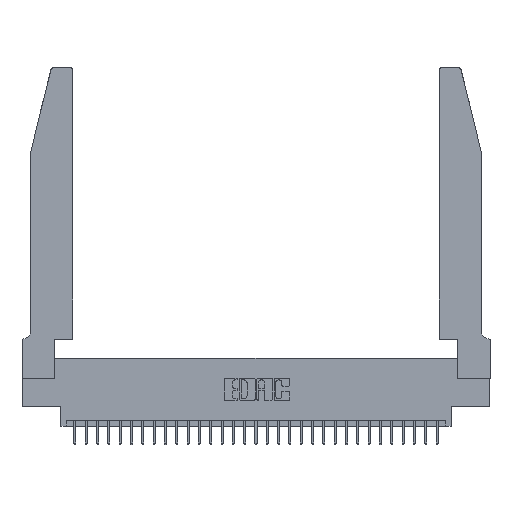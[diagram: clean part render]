
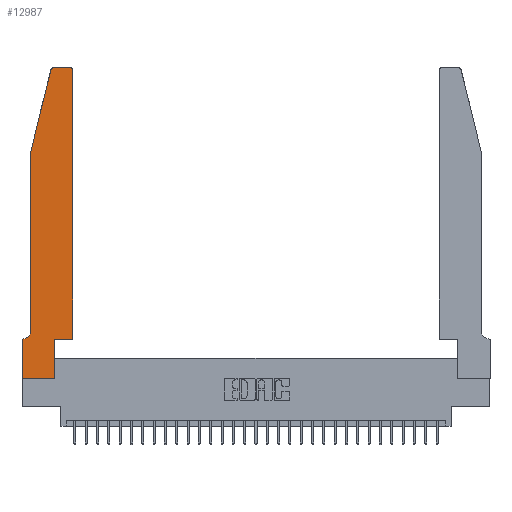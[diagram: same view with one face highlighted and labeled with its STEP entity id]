
A CAD part, top view. The second image highlights one B-rep face of the part: STEP entity #12987.
In plain terms, the highlighted planar face has unit normal (0, 0, 1).
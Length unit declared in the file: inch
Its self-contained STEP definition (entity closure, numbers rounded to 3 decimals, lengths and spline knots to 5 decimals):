
#38 = DIRECTION ( 'NONE',  ( 1., 0., 0. ) ) ;
#289 = EDGE_CURVE ( 'NONE', #4363, #17346, #24112, .T. ) ;
#447 = VERTEX_POINT ( 'NONE', #28399 ) ;
#587 = EDGE_LOOP ( 'NONE', ( #31960, #29077, #23572, #21709, #996, #9938, #24068, #21343, #4965, #27553, #31912, #23600 ) ) ;
#854 = VERTEX_POINT ( 'NONE', #930 ) ;
#930 = CARTESIAN_POINT ( 'NONE',  ( 0., 0.35, 0.37 ) ) ;
#996 = ORIENTED_EDGE ( 'NONE', *, *, #19184, .T. ) ;
#1919 = VERTEX_POINT ( 'NONE', #4878 ) ;
#2637 = CARTESIAN_POINT ( 'NONE',  ( 0.284, 2.72, 0.37 ) ) ;
#2673 = EDGE_CURVE ( 'NONE', #9499, #854, #15958, .T. ) ;
#2981 = CARTESIAN_POINT ( 'NONE',  ( 0.2865, 0.35, 0.37 ) ) ;
#3252 = CARTESIAN_POINT ( 'NONE',  ( 0.0755, 2., 0.37 ) ) ;
#4006 = CARTESIAN_POINT ( 'NONE',  ( 0.0755, 0.42, 0.37 ) ) ;
#4363 = VERTEX_POINT ( 'NONE', #11762 ) ;
#4402 = VECTOR ( 'NONE', #19186, 39.37008 ) ;
#4539 = LINE ( 'NONE', #12623, #24396 ) ;
#4878 = CARTESIAN_POINT ( 'NONE',  ( 0.284, 2.75, 0.37 ) ) ;
#4938 = CARTESIAN_POINT ( 'NONE',  ( 0.4505, 0.35, 0.37 ) ) ;
#4944 = CARTESIAN_POINT ( 'NONE',  ( 0., 0., 0.37 ) ) ;
#4965 = ORIENTED_EDGE ( 'NONE', *, *, #21294, .T. ) ;
#5196 = DIRECTION ( 'NONE',  ( 1., 0., 0. ) ) ;
#5439 = CARTESIAN_POINT ( 'NONE',  ( 0.25487, 2.72718, 0.37 ) ) ;
#5756 = VERTEX_POINT ( 'NONE', #14780 ) ;
#6135 = CIRCLE ( 'NONE', #13825, 0.03 ) ;
#6938 = EDGE_CURVE ( 'NONE', #13490, #1919, #31354, .T. ) ;
#6968 = VERTEX_POINT ( 'NONE', #4944 ) ;
#7221 = EDGE_CURVE ( 'NONE', #854, #6968, #30202, .T. ) ;
#7657 = LINE ( 'NONE', #10532, #20127 ) ;
#7766 = EDGE_CURVE ( 'NONE', #6968, #19508, #7657, .T. ) ;
#8386 = CARTESIAN_POINT ( 'NONE',  ( 0., 0., 0.37 ) ) ;
#8520 = VECTOR ( 'NONE', #12875, 39.37008 ) ;
#8575 = EDGE_CURVE ( 'NONE', #447, #13490, #12321, .T. ) ;
#8861 = CARTESIAN_POINT ( 'NONE',  ( 0.4205, 2.72, 0.37 ) ) ;
#9201 = CARTESIAN_POINT ( 'NONE',  ( 0.4505, 0.35, 0.37 ) ) ;
#9499 = VERTEX_POINT ( 'NONE', #24475 ) ;
#9886 = CARTESIAN_POINT ( 'NONE',  ( 0.4205, 2.75, 0.37 ) ) ;
#9938 = ORIENTED_EDGE ( 'NONE', *, *, #2673, .T. ) ;
#10344 = DIRECTION ( 'NONE',  ( 0., 0., -1. ) ) ;
#10532 = CARTESIAN_POINT ( 'NONE',  ( 0., 0., 0.37 ) ) ;
#11118 = LINE ( 'NONE', #9201, #4402 ) ;
#11346 = DIRECTION ( 'NONE',  ( 1., 0., 0. ) ) ;
#11762 = CARTESIAN_POINT ( 'NONE',  ( 0.2865, 0.35, 0.37 ) ) ;
#11779 = AXIS2_PLACEMENT_3D ( 'NONE', #25109, #10344, #27546 ) ;
#11799 = VECTOR ( 'NONE', #17349, 39.37008 ) ;
#12321 = CIRCLE ( 'NONE', #32066, 0.03 ) ;
#12333 = AXIS2_PLACEMENT_3D ( 'NONE', #27349, #15184, #38 ) ;
#12623 = CARTESIAN_POINT ( 'NONE',  ( 0.0755, 2., 0.37 ) ) ;
#12651 = PLANE ( 'NONE',  #12333 ) ;
#12875 = DIRECTION ( 'NONE',  ( -1., 0., 0. ) ) ;
#12987 = ADVANCED_FACE ( 'NONE', ( #25941 ), #12651, .T. ) ;
#13184 = EDGE_CURVE ( 'NONE', #5756, #17827, #14042, .T. ) ;
#13195 = DIRECTION ( 'NONE',  ( 1., 0., 0. ) ) ;
#13490 = VERTEX_POINT ( 'NONE', #9886 ) ;
#13540 = EDGE_CURVE ( 'NONE', #13645, #5756, #4539, .T. ) ;
#13645 = VERTEX_POINT ( 'NONE', #5439 ) ;
#13825 = AXIS2_PLACEMENT_3D ( 'NONE', #2637, #20164, #5196 ) ;
#14042 = LINE ( 'NONE', #3252, #26310 ) ;
#14238 = EDGE_CURVE ( 'NONE', #1919, #13645, #6135, .T. ) ;
#14780 = CARTESIAN_POINT ( 'NONE',  ( 0.0755, 2., 0.37 ) ) ;
#15184 = DIRECTION ( 'NONE',  ( 0., 0., 1. ) ) ;
#15958 = LINE ( 'NONE', #22702, #8520 ) ;
#16527 = EDGE_CURVE ( 'NONE', #17346, #447, #11118, .T. ) ;
#17263 = VECTOR ( 'NONE', #28093, 39.37008 ) ;
#17346 = VERTEX_POINT ( 'NONE', #24598 ) ;
#17349 = DIRECTION ( 'NONE',  ( -1., 0., 0. ) ) ;
#17456 = VECTOR ( 'NONE', #18009, 39.37008 ) ;
#17827 = VERTEX_POINT ( 'NONE', #4006 ) ;
#18009 = DIRECTION ( 'NONE',  ( 0., 1., 0. ) ) ;
#18024 = DIRECTION ( 'NONE',  ( 1., 0., 0. ) ) ;
#19184 = EDGE_CURVE ( 'NONE', #17827, #9499, #22569, .T. ) ;
#19186 = DIRECTION ( 'NONE',  ( 0., 1., 0. ) ) ;
#19508 = VERTEX_POINT ( 'NONE', #21375 ) ;
#20127 = VECTOR ( 'NONE', #18024, 39.37008 ) ;
#20164 = DIRECTION ( 'NONE',  ( 0., 0., 1. ) ) ;
#21294 = EDGE_CURVE ( 'NONE', #19508, #4363, #30383, .T. ) ;
#21343 = ORIENTED_EDGE ( 'NONE', *, *, #7766, .T. ) ;
#21375 = CARTESIAN_POINT ( 'NONE',  ( 0.2865, 0., 0.37 ) ) ;
#21709 = ORIENTED_EDGE ( 'NONE', *, *, #13184, .T. ) ;
#22569 = CIRCLE ( 'NONE', #11779, 0.07 ) ;
#22702 = CARTESIAN_POINT ( 'NONE',  ( 0.0755, 0.35, 0.37 ) ) ;
#23572 = ORIENTED_EDGE ( 'NONE', *, *, #13540, .T. ) ;
#23600 = ORIENTED_EDGE ( 'NONE', *, *, #8575, .T. ) ;
#24068 = ORIENTED_EDGE ( 'NONE', *, *, #7221, .T. ) ;
#24112 = LINE ( 'NONE', #4938, #29765 ) ;
#24396 = VECTOR ( 'NONE', #29752, 39.37008 ) ;
#24475 = CARTESIAN_POINT ( 'NONE',  ( 0.0055, 0.35, 0.37 ) ) ;
#24598 = CARTESIAN_POINT ( 'NONE',  ( 0.4505, 0.35, 0.37 ) ) ;
#25109 = CARTESIAN_POINT ( 'NONE',  ( 0.0055, 0.42, 0.37 ) ) ;
#25941 = FACE_OUTER_BOUND ( 'NONE', #587, .T. ) ;
#26115 = DIRECTION ( 'NONE',  ( 0., 0., 1. ) ) ;
#26310 = VECTOR ( 'NONE', #27968, 39.37008 ) ;
#27057 = CARTESIAN_POINT ( 'NONE',  ( 0.2605, 2.75, 0.37 ) ) ;
#27349 = CARTESIAN_POINT ( 'NONE',  ( 0., 0.35, 0.37 ) ) ;
#27546 = DIRECTION ( 'NONE',  ( -1., 0., 0. ) ) ;
#27553 = ORIENTED_EDGE ( 'NONE', *, *, #289, .T. ) ;
#27968 = DIRECTION ( 'NONE',  ( 0., -1., 0. ) ) ;
#28093 = DIRECTION ( 'NONE',  ( 0., -1., 0. ) ) ;
#28399 = CARTESIAN_POINT ( 'NONE',  ( 0.4505, 2.72, 0.37 ) ) ;
#29077 = ORIENTED_EDGE ( 'NONE', *, *, #14238, .T. ) ;
#29752 = DIRECTION ( 'NONE',  ( -0.239, -0.971, 0. ) ) ;
#29765 = VECTOR ( 'NONE', #13195, 39.37008 ) ;
#30202 = LINE ( 'NONE', #8386, #17263 ) ;
#30383 = LINE ( 'NONE', #2981, #17456 ) ;
#31354 = LINE ( 'NONE', #27057, #11799 ) ;
#31912 = ORIENTED_EDGE ( 'NONE', *, *, #16527, .T. ) ;
#31960 = ORIENTED_EDGE ( 'NONE', *, *, #6938, .T. ) ;
#32066 = AXIS2_PLACEMENT_3D ( 'NONE', #8861, #26115, #11346 ) ;
